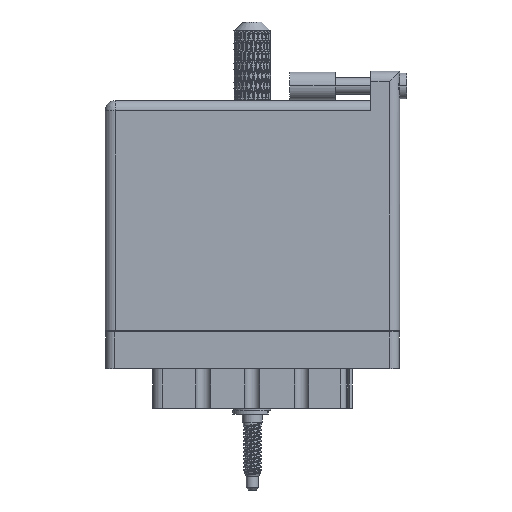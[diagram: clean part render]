
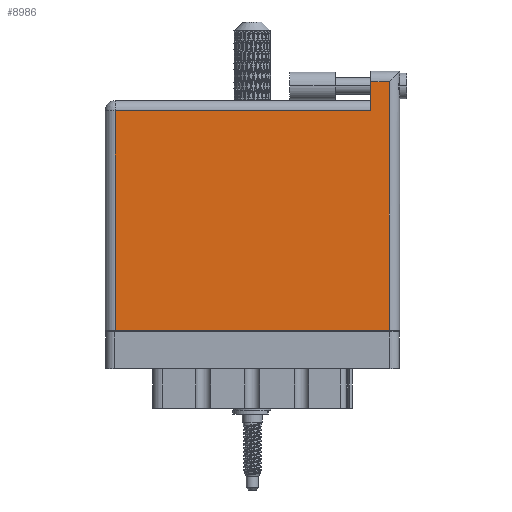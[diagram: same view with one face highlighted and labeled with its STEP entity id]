
A CAD part, front view. The second image highlights one B-rep face of the part: STEP entity #8986.
In plain terms, the highlighted face is planar.
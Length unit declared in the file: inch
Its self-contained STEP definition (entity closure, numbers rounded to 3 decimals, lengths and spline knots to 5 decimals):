
#4130 = LINE ( 'NONE', #97043, #37573 ) ;
#5474 = DIRECTION ( 'NONE',  ( 0., 1., 0. ) ) ;
#7091 = VERTEX_POINT ( 'NONE', #103219 ) ;
#8082 = LINE ( 'NONE', #86621, #68582 ) ;
#8986 = ADVANCED_FACE ( 'NONE', ( #32993 ), #27525, .F. ) ;
#10589 = VECTOR ( 'NONE', #65170, 39.37008 ) ;
#10611 = VERTEX_POINT ( 'NONE', #12066 ) ;
#10811 = DIRECTION ( 'NONE',  ( -1., 0., 0. ) ) ;
#11389 = DIRECTION ( 'NONE',  ( -1., 0., 0. ) ) ;
#12066 = CARTESIAN_POINT ( 'NONE',  ( 0.07, 1.496, 0. ) ) ;
#14431 = LINE ( 'NONE', #88288, #10589 ) ;
#18408 = EDGE_CURVE ( 'NONE', #7091, #80756, #14431, .T. ) ;
#20721 = ORIENTED_EDGE ( 'NONE', *, *, #70167, .T. ) ;
#21341 = DIRECTION ( 'NONE',  ( 0., -1., 0. ) ) ;
#27438 = VERTEX_POINT ( 'NONE', #96932 ) ;
#27525 = PLANE ( 'NONE',  #63136 ) ;
#28824 = ORIENTED_EDGE ( 'NONE', *, *, #59321, .T. ) ;
#32993 = FACE_OUTER_BOUND ( 'NONE', #64553, .T. ) ;
#34192 = DIRECTION ( 'NONE',  ( 0., -1., 0. ) ) ;
#35136 = EDGE_CURVE ( 'NONE', #80756, #47408, #83628, .T. ) ;
#37573 = VECTOR ( 'NONE', #46579, 39.37008 ) ;
#39444 = ORIENTED_EDGE ( 'NONE', *, *, #18408, .T. ) ;
#44678 = ORIENTED_EDGE ( 'NONE', *, *, #35136, .T. ) ;
#45149 = LINE ( 'NONE', #105572, #64505 ) ;
#46579 = DIRECTION ( 'NONE',  ( 1., 0., 0. ) ) ;
#47256 = CARTESIAN_POINT ( 'NONE',  ( 1.811, 1.696, 0. ) ) ;
#47408 = VERTEX_POINT ( 'NONE', #68789 ) ;
#47898 = VERTEX_POINT ( 'NONE', #87746 ) ;
#48469 = LINE ( 'NONE', #60153, #67802 ) ;
#51454 = CARTESIAN_POINT ( 'NONE',  ( 1.811, 1.766, 0. ) ) ;
#59119 = VECTOR ( 'NONE', #34192, 39.37008 ) ;
#59321 = EDGE_CURVE ( 'NONE', #47898, #27438, #4130, .T. ) ;
#59326 = ORIENTED_EDGE ( 'NONE', *, *, #71635, .T. ) ;
#60153 = CARTESIAN_POINT ( 'NONE',  ( 0., 1.496, 0. ) ) ;
#62532 = CARTESIAN_POINT ( 'NONE',  ( 0., 1.566, 0. ) ) ;
#63136 = AXIS2_PLACEMENT_3D ( 'NONE', #62532, #79160, #11389 ) ;
#64505 = VECTOR ( 'NONE', #5474, 39.37008 ) ;
#64553 = EDGE_LOOP ( 'NONE', ( #28824, #59326, #39444, #44678, #71733, #20721 ) ) ;
#65170 = DIRECTION ( 'NONE',  ( -1., 0., 0. ) ) ;
#67802 = VECTOR ( 'NONE', #10811, 39.37008 ) ;
#68582 = VECTOR ( 'NONE', #21341, 39.37008 ) ;
#68789 = CARTESIAN_POINT ( 'NONE',  ( 1.811, 1.496, 0. ) ) ;
#70167 = EDGE_CURVE ( 'NONE', #10611, #47898, #8082, .T. ) ;
#71635 = EDGE_CURVE ( 'NONE', #27438, #7091, #45149, .T. ) ;
#71733 = ORIENTED_EDGE ( 'NONE', *, *, #75248, .T. ) ;
#75248 = EDGE_CURVE ( 'NONE', #47408, #10611, #48469, .T. ) ;
#79160 = DIRECTION ( 'NONE',  ( 0., 0., -1. ) ) ;
#80756 = VERTEX_POINT ( 'NONE', #47256 ) ;
#83628 = LINE ( 'NONE', #51454, #59119 ) ;
#86621 = CARTESIAN_POINT ( 'NONE',  ( 0.07, 0., 0. ) ) ;
#87746 = CARTESIAN_POINT ( 'NONE',  ( 0.07, 0., 0. ) ) ;
#88288 = CARTESIAN_POINT ( 'NONE',  ( 0., 1.696, 0. ) ) ;
#96932 = CARTESIAN_POINT ( 'NONE',  ( 1.938, 0., 0. ) ) ;
#97043 = CARTESIAN_POINT ( 'NONE',  ( 0., 0., 0. ) ) ;
#103219 = CARTESIAN_POINT ( 'NONE',  ( 1.938, 1.696, 0. ) ) ;
#105572 = CARTESIAN_POINT ( 'NONE',  ( 1.938, 1.766, 0. ) ) ;
